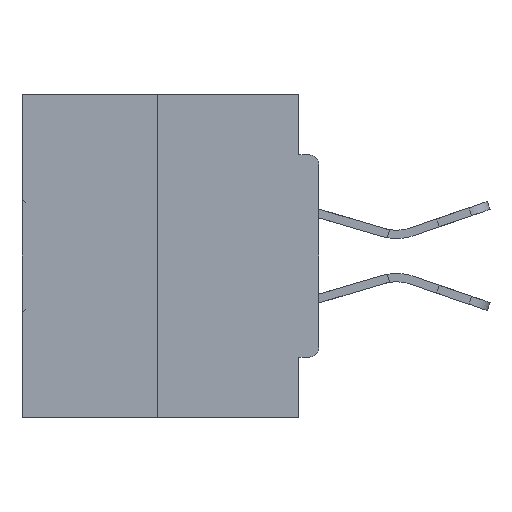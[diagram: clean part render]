
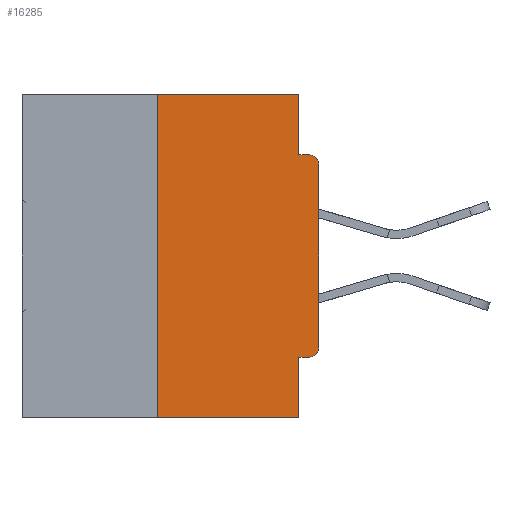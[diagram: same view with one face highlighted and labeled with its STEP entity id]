
A CAD part, left-side view. The second image highlights one B-rep face of the part: STEP entity #16285.
In plain terms, the highlighted planar face has unit normal (-1, 0, 0).
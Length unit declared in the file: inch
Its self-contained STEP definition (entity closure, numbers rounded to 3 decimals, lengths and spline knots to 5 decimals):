
#54 = LINE ( 'NONE', #4139, #39709 ) ;
#2966 = ORIENTED_EDGE ( 'NONE', *, *, #42684, .F. ) ;
#3655 = EDGE_CURVE ( 'NONE', #22856, #42873, #22644, .T. ) ;
#4139 = CARTESIAN_POINT ( 'NONE',  ( 0., 0.25, 0. ) ) ;
#4793 = CARTESIAN_POINT ( 'NONE',  ( 0., 0., -0.0935 ) ) ;
#6735 = ORIENTED_EDGE ( 'NONE', *, *, #41506, .F. ) ;
#6810 = CARTESIAN_POINT ( 'NONE',  ( 0., 0.031, -0.0935 ) ) ;
#7430 = VERTEX_POINT ( 'NONE', #12901 ) ;
#7451 = EDGE_CURVE ( 'NONE', #40546, #42873, #33262, .T. ) ;
#7777 = VECTOR ( 'NONE', #21541, 39.37008 ) ;
#8642 = ORIENTED_EDGE ( 'NONE', *, *, #16922, .F. ) ;
#9587 = LINE ( 'NONE', #13800, #36512 ) ;
#10165 = VECTOR ( 'NONE', #29376, 39.37008 ) ;
#10496 = ORIENTED_EDGE ( 'NONE', *, *, #17391, .T. ) ;
#11331 = CIRCLE ( 'NONE', #16882, 0.015 ) ;
#12394 = CARTESIAN_POINT ( 'NONE',  ( 0., 0.015, -0.0935 ) ) ;
#12520 = CARTESIAN_POINT ( 'NONE',  ( 0., 0.031, -0.4065 ) ) ;
#12755 = DIRECTION ( 'NONE',  ( 0., -1., 0. ) ) ;
#12901 = CARTESIAN_POINT ( 'NONE',  ( 0., 0.25, 0. ) ) ;
#12968 = VECTOR ( 'NONE', #12755, 39.37008 ) ;
#12984 = VERTEX_POINT ( 'NONE', #6810 ) ;
#13800 = CARTESIAN_POINT ( 'NONE',  ( 0., 0., 0. ) ) ;
#14111 = CARTESIAN_POINT ( 'NONE',  ( 0., 0.46, 0. ) ) ;
#14261 = DIRECTION ( 'NONE',  ( 0., 0., 1. ) ) ;
#14545 = CARTESIAN_POINT ( 'NONE',  ( 0., 0.015, -0.3915 ) ) ;
#14592 = PLANE ( 'NONE',  #21086 ) ;
#15255 = ORIENTED_EDGE ( 'NONE', *, *, #7451, .T. ) ;
#15475 = EDGE_LOOP ( 'NONE', ( #8642, #2966, #15255, #21846, #44746, #23398, #10496, #27916, #21130, #6735 ) ) ;
#15653 = VERTEX_POINT ( 'NONE', #12394 ) ;
#16187 = CARTESIAN_POINT ( 'NONE',  ( 0., 0.46, 0. ) ) ;
#16229 = DIRECTION ( 'NONE',  ( 0., 1., 0. ) ) ;
#16285 = ADVANCED_FACE ( 'NONE', ( #20095 ), #14592, .F. ) ;
#16452 = EDGE_CURVE ( 'NONE', #16728, #15653, #17349, .T. ) ;
#16728 = VERTEX_POINT ( 'NONE', #21605 ) ;
#16882 = AXIS2_PLACEMENT_3D ( 'NONE', #14545, #36036, #18102 ) ;
#16922 = EDGE_CURVE ( 'NONE', #7430, #18300, #36554, .T. ) ;
#17040 = CARTESIAN_POINT ( 'NONE',  ( 0., 0.015, -0.1085 ) ) ;
#17349 = CIRCLE ( 'NONE', #31045, 0.015 ) ;
#17391 = EDGE_CURVE ( 'NONE', #37679, #16728, #9587, .T. ) ;
#17685 = DIRECTION ( 'NONE',  ( 1., 0., 0. ) ) ;
#18028 = CARTESIAN_POINT ( 'NONE',  ( 0., 0.031, -0.5 ) ) ;
#18102 = DIRECTION ( 'NONE',  ( 0., 0., -1. ) ) ;
#18133 = DIRECTION ( 'NONE',  ( 0., 0., -1. ) ) ;
#18300 = VERTEX_POINT ( 'NONE', #38841 ) ;
#19288 = VECTOR ( 'NONE', #16229, 39.37008 ) ;
#19597 = CARTESIAN_POINT ( 'NONE',  ( 0., 0., -0.4065 ) ) ;
#20050 = EDGE_CURVE ( 'NONE', #44348, #22856, #43956, .T. ) ;
#20095 = FACE_OUTER_BOUND ( 'NONE', #15475, .T. ) ;
#20547 = DIRECTION ( 'NONE',  ( -1., 0., 0. ) ) ;
#21086 = AXIS2_PLACEMENT_3D ( 'NONE', #14111, #17685, #39160 ) ;
#21130 = ORIENTED_EDGE ( 'NONE', *, *, #35260, .F. ) ;
#21541 = DIRECTION ( 'NONE',  ( 0., 0., -1. ) ) ;
#21605 = CARTESIAN_POINT ( 'NONE',  ( 0., 0., -0.1085 ) ) ;
#21846 = ORIENTED_EDGE ( 'NONE', *, *, #3655, .F. ) ;
#22644 = LINE ( 'NONE', #18028, #7777 ) ;
#22856 = VERTEX_POINT ( 'NONE', #12520 ) ;
#23398 = ORIENTED_EDGE ( 'NONE', *, *, #34486, .T. ) ;
#25077 = DIRECTION ( 'NONE',  ( 0., 0., 1. ) ) ;
#26586 = DIRECTION ( 'NONE',  ( 0., -1., 0. ) ) ;
#26614 = VECTOR ( 'NONE', #18133, 39.37008 ) ;
#26851 = CARTESIAN_POINT ( 'NONE',  ( 0., 0.031, -0.5 ) ) ;
#27916 = ORIENTED_EDGE ( 'NONE', *, *, #16452, .T. ) ;
#29376 = DIRECTION ( 'NONE',  ( 0., -1., 0. ) ) ;
#30927 = CARTESIAN_POINT ( 'NONE',  ( 0., 0.25, -0.5 ) ) ;
#31045 = AXIS2_PLACEMENT_3D ( 'NONE', #17040, #20547, #42023 ) ;
#33262 = LINE ( 'NONE', #37024, #12968 ) ;
#34486 = EDGE_CURVE ( 'NONE', #44348, #37679, #11331, .T. ) ;
#35260 = EDGE_CURVE ( 'NONE', #12984, #15653, #37093, .T. ) ;
#36036 = DIRECTION ( 'NONE',  ( -1., 0., 0. ) ) ;
#36040 = CARTESIAN_POINT ( 'NONE',  ( 0., 0., -0.3915 ) ) ;
#36512 = VECTOR ( 'NONE', #14261, 39.37008 ) ;
#36554 = LINE ( 'NONE', #16187, #40384 ) ;
#37024 = CARTESIAN_POINT ( 'NONE',  ( 0., 0.46, -0.5 ) ) ;
#37093 = LINE ( 'NONE', #4793, #10165 ) ;
#37679 = VERTEX_POINT ( 'NONE', #36040 ) ;
#38841 = CARTESIAN_POINT ( 'NONE',  ( 0., 0.031, 0. ) ) ;
#39160 = DIRECTION ( 'NONE',  ( 0., 0., -1. ) ) ;
#39709 = VECTOR ( 'NONE', #25077, 39.37008 ) ;
#39840 = LINE ( 'NONE', #42327, #26614 ) ;
#40384 = VECTOR ( 'NONE', #26586, 39.37008 ) ;
#40546 = VERTEX_POINT ( 'NONE', #30927 ) ;
#41506 = EDGE_CURVE ( 'NONE', #18300, #12984, #39840, .T. ) ;
#42023 = DIRECTION ( 'NONE',  ( 0., 0., -1. ) ) ;
#42139 = CARTESIAN_POINT ( 'NONE',  ( 0., 0.015, -0.4065 ) ) ;
#42327 = CARTESIAN_POINT ( 'NONE',  ( 0., 0.031, 0. ) ) ;
#42684 = EDGE_CURVE ( 'NONE', #40546, #7430, #54, .T. ) ;
#42873 = VERTEX_POINT ( 'NONE', #26851 ) ;
#43956 = LINE ( 'NONE', #19597, #19288 ) ;
#44348 = VERTEX_POINT ( 'NONE', #42139 ) ;
#44746 = ORIENTED_EDGE ( 'NONE', *, *, #20050, .F. ) ;
